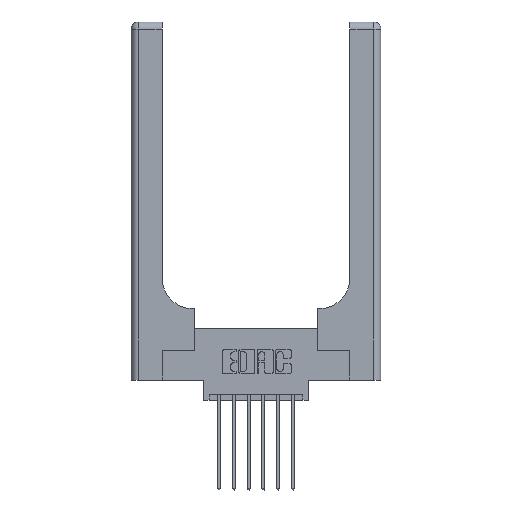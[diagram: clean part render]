
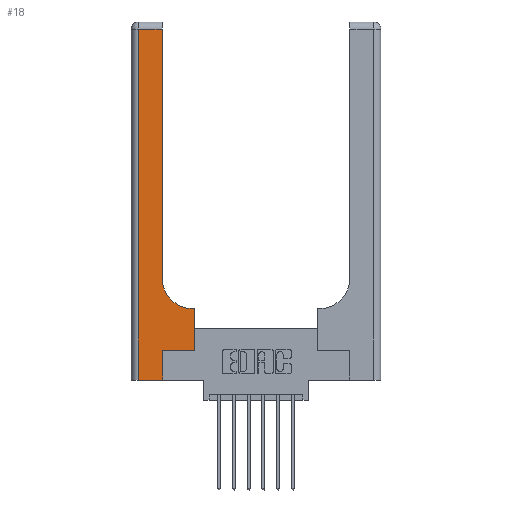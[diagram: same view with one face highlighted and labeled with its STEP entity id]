
A CAD part, top view. The second image highlights one B-rep face of the part: STEP entity #18.
In plain terms, the highlighted planar face has unit normal (0, 0, 1).
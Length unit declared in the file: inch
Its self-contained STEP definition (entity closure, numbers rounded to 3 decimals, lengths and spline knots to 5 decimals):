
#18 = ADVANCED_FACE ( 'NONE', ( #13842 ), #2018, .F. ) ;
#196 = ORIENTED_EDGE ( 'NONE', *, *, #1288, .T. ) ;
#318 = CIRCLE ( 'NONE', #9237, 0.25 ) ;
#339 = DIRECTION ( 'NONE',  ( 0., 1., 0. ) ) ;
#647 = CARTESIAN_POINT ( 'NONE',  ( 0.26, 0.85, 0.37 ) ) ;
#672 = DIRECTION ( 'NONE',  ( 0., 0., -1. ) ) ;
#704 = CARTESIAN_POINT ( 'NONE',  ( 0., 2.94, 0.37 ) ) ;
#952 = AXIS2_PLACEMENT_3D ( 'NONE', #2062, #1953, #1937 ) ;
#1288 = EDGE_CURVE ( 'NONE', #5455, #3539, #6462, .T. ) ;
#1328 = LINE ( 'NONE', #7742, #12532 ) ;
#1449 = CARTESIAN_POINT ( 'NONE',  ( 0.26, 3., 0.37 ) ) ;
#1937 = DIRECTION ( 'NONE',  ( -1., 0., 0. ) ) ;
#1953 = DIRECTION ( 'NONE',  ( 0., 0., -1. ) ) ;
#2018 = PLANE ( 'NONE',  #952 ) ;
#2062 = CARTESIAN_POINT ( 'NONE',  ( 0., 3., 0.37 ) ) ;
#2186 = EDGE_CURVE ( 'NONE', #11393, #5455, #4579, .T. ) ;
#3507 = CARTESIAN_POINT ( 'NONE',  ( 0.265, 0., 0.37 ) ) ;
#3539 = VERTEX_POINT ( 'NONE', #8602 ) ;
#3594 = VECTOR ( 'NONE', #6087, 39.37008 ) ;
#3759 = CARTESIAN_POINT ( 'NONE',  ( 0.51, 0.6, 0.37 ) ) ;
#3981 = ORIENTED_EDGE ( 'NONE', *, *, #7298, .T. ) ;
#4430 = CARTESIAN_POINT ( 'NONE',  ( 0.06, 0., 0.37 ) ) ;
#4448 = CARTESIAN_POINT ( 'NONE',  ( 0.26, 2.94, 0.37 ) ) ;
#4537 = DIRECTION ( 'NONE',  ( 0., 1., 0. ) ) ;
#4579 = LINE ( 'NONE', #6392, #8499 ) ;
#4594 = ORIENTED_EDGE ( 'NONE', *, *, #11893, .T. ) ;
#4608 = LINE ( 'NONE', #3507, #6809 ) ;
#4827 = VERTEX_POINT ( 'NONE', #4448 ) ;
#4859 = EDGE_CURVE ( 'NONE', #7622, #7816, #11961, .T. ) ;
#5287 = LINE ( 'NONE', #1449, #10375 ) ;
#5383 = ORIENTED_EDGE ( 'NONE', *, *, #4859, .T. ) ;
#5455 = VERTEX_POINT ( 'NONE', #4430 ) ;
#5590 = DIRECTION ( 'NONE',  ( -1., 0., 0. ) ) ;
#5807 = LINE ( 'NONE', #6131, #8373 ) ;
#6086 = CARTESIAN_POINT ( 'NONE',  ( 0.06, 2.94, 0.37 ) ) ;
#6087 = DIRECTION ( 'NONE',  ( 1., 0., 0. ) ) ;
#6124 = VERTEX_POINT ( 'NONE', #647 ) ;
#6131 = CARTESIAN_POINT ( 'NONE',  ( 0.265, 0.25, 0.37 ) ) ;
#6286 = EDGE_LOOP ( 'NONE', ( #8151, #3981, #13108, #196, #7406, #13189, #5383, #12687, #4594 ) ) ;
#6392 = CARTESIAN_POINT ( 'NONE',  ( 0.06, 3., 0.37 ) ) ;
#6456 = CARTESIAN_POINT ( 'NONE',  ( 0.265, 0.25, 0.37 ) ) ;
#6462 = LINE ( 'NONE', #11466, #3594 ) ;
#6592 = VERTEX_POINT ( 'NONE', #3759 ) ;
#6809 = VECTOR ( 'NONE', #8965, 39.37008 ) ;
#7214 = CARTESIAN_POINT ( 'NONE',  ( 0.51, 0.85, 0.37 ) ) ;
#7247 = DIRECTION ( 'NONE',  ( -1., 0., 0. ) ) ;
#7298 = EDGE_CURVE ( 'NONE', #4827, #11393, #11894, .T. ) ;
#7406 = ORIENTED_EDGE ( 'NONE', *, *, #12287, .T. ) ;
#7622 = VERTEX_POINT ( 'NONE', #12185 ) ;
#7742 = CARTESIAN_POINT ( 'NONE',  ( 0.26, 0.6, 0.37 ) ) ;
#7816 = VERTEX_POINT ( 'NONE', #9503 ) ;
#8151 = ORIENTED_EDGE ( 'NONE', *, *, #11728, .T. ) ;
#8323 = DIRECTION ( 'NONE',  ( 1., 0., 0. ) ) ;
#8373 = VECTOR ( 'NONE', #12606, 39.37008 ) ;
#8499 = VECTOR ( 'NONE', #13971, 39.37008 ) ;
#8602 = CARTESIAN_POINT ( 'NONE',  ( 0.265, 0., 0.37 ) ) ;
#8965 = DIRECTION ( 'NONE',  ( 0., 1., 0. ) ) ;
#9043 = VECTOR ( 'NONE', #7247, 39.37008 ) ;
#9237 = AXIS2_PLACEMENT_3D ( 'NONE', #7214, #672, #8323 ) ;
#9503 = CARTESIAN_POINT ( 'NONE',  ( 0.528, 0.6, 0.37 ) ) ;
#10375 = VECTOR ( 'NONE', #339, 39.37008 ) ;
#11393 = VERTEX_POINT ( 'NONE', #6086 ) ;
#11412 = EDGE_CURVE ( 'NONE', #13337, #7622, #5807, .T. ) ;
#11466 = CARTESIAN_POINT ( 'NONE',  ( 0., 0., 0.37 ) ) ;
#11622 = VECTOR ( 'NONE', #4537, 39.37008 ) ;
#11728 = EDGE_CURVE ( 'NONE', #6124, #4827, #5287, .T. ) ;
#11893 = EDGE_CURVE ( 'NONE', #6592, #6124, #318, .T. ) ;
#11894 = LINE ( 'NONE', #704, #9043 ) ;
#11961 = LINE ( 'NONE', #12084, #11622 ) ;
#12084 = CARTESIAN_POINT ( 'NONE',  ( 0.528, 0.25, 0.37 ) ) ;
#12185 = CARTESIAN_POINT ( 'NONE',  ( 0.528, 0.25, 0.37 ) ) ;
#12287 = EDGE_CURVE ( 'NONE', #3539, #13337, #4608, .T. ) ;
#12532 = VECTOR ( 'NONE', #5590, 39.37008 ) ;
#12606 = DIRECTION ( 'NONE',  ( 1., 0., 0. ) ) ;
#12687 = ORIENTED_EDGE ( 'NONE', *, *, #13502, .T. ) ;
#13108 = ORIENTED_EDGE ( 'NONE', *, *, #2186, .T. ) ;
#13189 = ORIENTED_EDGE ( 'NONE', *, *, #11412, .T. ) ;
#13337 = VERTEX_POINT ( 'NONE', #6456 ) ;
#13502 = EDGE_CURVE ( 'NONE', #7816, #6592, #1328, .T. ) ;
#13842 = FACE_OUTER_BOUND ( 'NONE', #6286, .T. ) ;
#13971 = DIRECTION ( 'NONE',  ( 0., -1., 0. ) ) ;
